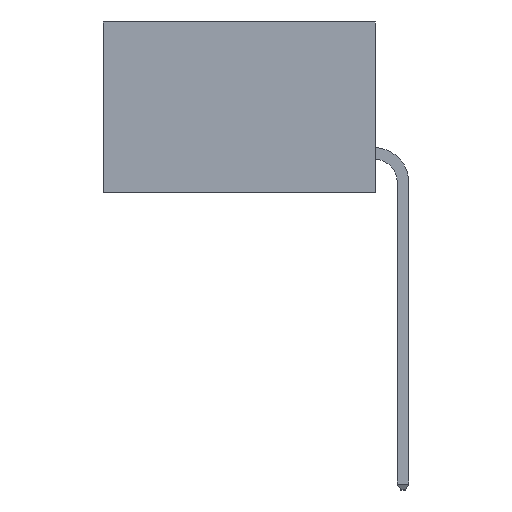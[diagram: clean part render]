
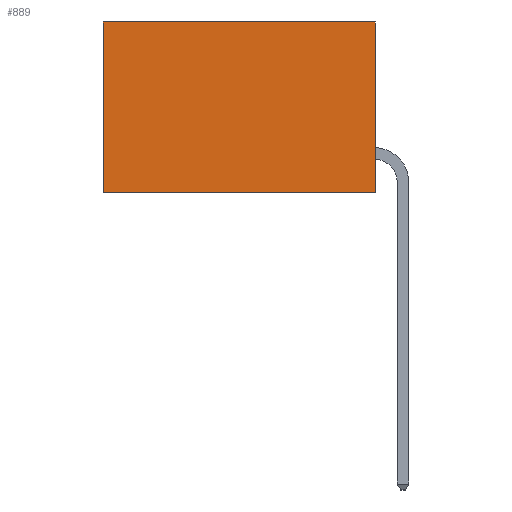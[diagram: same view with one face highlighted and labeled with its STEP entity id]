
A CAD part, left-side view. The second image highlights one B-rep face of the part: STEP entity #889.
In plain terms, the highlighted planar face has unit normal (-1, 0, 0).
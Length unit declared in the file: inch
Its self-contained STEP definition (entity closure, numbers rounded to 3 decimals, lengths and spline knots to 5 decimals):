
#247 = ORIENTED_EDGE ( 'NONE', *, *, #2209, .F. ) ;
#285 = ORIENTED_EDGE ( 'NONE', *, *, #8648, .F. ) ;
#499 = CARTESIAN_POINT ( 'NONE',  ( 0.277, 0.59, -0.37 ) ) ;
#533 = VECTOR ( 'NONE', #6534, 39.37008 ) ;
#818 = LINE ( 'NONE', #6570, #533 ) ;
#884 = VECTOR ( 'NONE', #9645, 39.37008 ) ;
#889 = ADVANCED_FACE ( 'NONE', ( #3035 ), #4936, .F. ) ;
#973 = ORIENTED_EDGE ( 'NONE', *, *, #8558, .T. ) ;
#1536 = VERTEX_POINT ( 'NONE', #2742 ) ;
#1620 = VERTEX_POINT ( 'NONE', #2863 ) ;
#2119 = VECTOR ( 'NONE', #7980, 39.37008 ) ;
#2209 = EDGE_CURVE ( 'NONE', #1536, #4278, #5328, .T. ) ;
#2742 = CARTESIAN_POINT ( 'NONE',  ( 0.277, 0., -0.37 ) ) ;
#2863 = CARTESIAN_POINT ( 'NONE',  ( 0.277, 0., 0. ) ) ;
#3035 = FACE_OUTER_BOUND ( 'NONE', #6094, .T. ) ;
#3238 = CARTESIAN_POINT ( 'NONE',  ( 0.277, 0.59, 0. ) ) ;
#3500 = AXIS2_PLACEMENT_3D ( 'NONE', #4674, #5302, #9298 ) ;
#3836 = VERTEX_POINT ( 'NONE', #3238 ) ;
#4278 = VERTEX_POINT ( 'NONE', #499 ) ;
#4446 = CARTESIAN_POINT ( 'NONE',  ( 0.277, 0., -0.37 ) ) ;
#4509 = DIRECTION ( 'NONE',  ( 0., 0., -1. ) ) ;
#4674 = CARTESIAN_POINT ( 'NONE',  ( 0.277, 0., -0.37 ) ) ;
#4936 = PLANE ( 'NONE',  #3500 ) ;
#5302 = DIRECTION ( 'NONE',  ( 1., 0., 0. ) ) ;
#5328 = LINE ( 'NONE', #9260, #884 ) ;
#5331 = CARTESIAN_POINT ( 'NONE',  ( 0.277, 0., 0. ) ) ;
#5786 = ORIENTED_EDGE ( 'NONE', *, *, #6348, .T. ) ;
#6094 = EDGE_LOOP ( 'NONE', ( #5786, #247, #285, #973 ) ) ;
#6348 = EDGE_CURVE ( 'NONE', #3836, #4278, #818, .T. ) ;
#6534 = DIRECTION ( 'NONE',  ( 0., 0., -1. ) ) ;
#6570 = CARTESIAN_POINT ( 'NONE',  ( 0.277, 0.59, -0.37 ) ) ;
#7412 = VECTOR ( 'NONE', #4509, 39.37008 ) ;
#7980 = DIRECTION ( 'NONE',  ( 0., 1., 0. ) ) ;
#8558 = EDGE_CURVE ( 'NONE', #1620, #3836, #10320, .T. ) ;
#8648 = EDGE_CURVE ( 'NONE', #1620, #1536, #9167, .T. ) ;
#9167 = LINE ( 'NONE', #4446, #7412 ) ;
#9260 = CARTESIAN_POINT ( 'NONE',  ( 0.277, 0., -0.37 ) ) ;
#9298 = DIRECTION ( 'NONE',  ( 0., 0., -1. ) ) ;
#9645 = DIRECTION ( 'NONE',  ( 0., 1., 0. ) ) ;
#10320 = LINE ( 'NONE', #5331, #2119 ) ;
